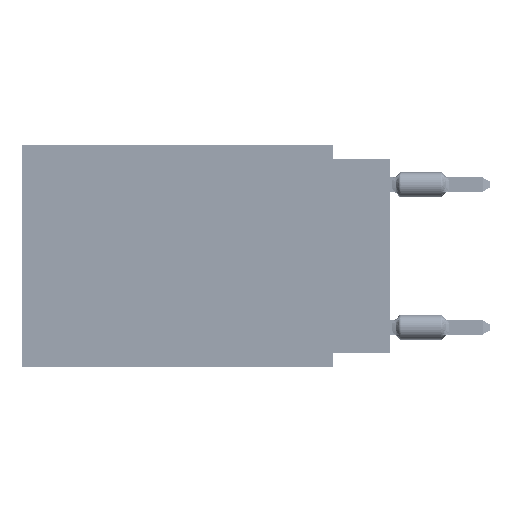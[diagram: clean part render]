
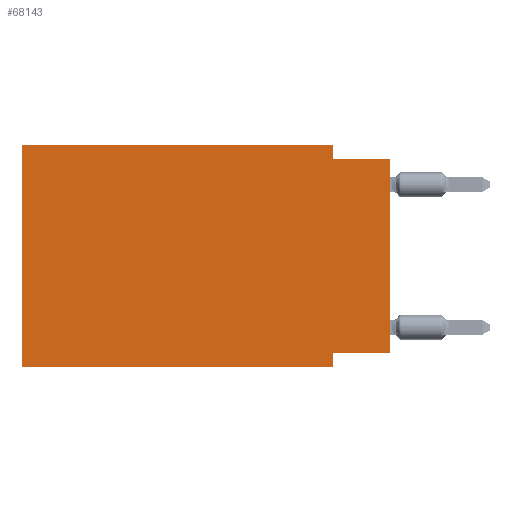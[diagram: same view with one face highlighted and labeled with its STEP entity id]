
A CAD part, left-side view. The second image highlights one B-rep face of the part: STEP entity #68143.
In plain terms, the highlighted planar face has unit normal (-1, 0, 0).
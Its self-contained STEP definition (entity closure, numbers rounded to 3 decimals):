
#1008 = CARTESIAN_POINT ( 'NONE',  ( 0., 16.383, -9.906 ) ) ;
#1446 = VERTEX_POINT ( 'NONE', #73461 ) ;
#2046 = CARTESIAN_POINT ( 'NONE',  ( 0., 16.383, 0. ) ) ;
#2713 = CARTESIAN_POINT ( 'NONE',  ( 0., 0., 0. ) ) ;
#3129 = DIRECTION ( 'NONE',  ( 0., 0., 1. ) ) ;
#3843 = EDGE_CURVE ( 'NONE', #80691, #40627, #19253, .T. ) ;
#4311 = VECTOR ( 'NONE', #3129, 1000. ) ;
#7272 = CARTESIAN_POINT ( 'NONE',  ( 0., 0., -9.271 ) ) ;
#7515 = DIRECTION ( 'NONE',  ( 0., -1., 0. ) ) ;
#8528 = VECTOR ( 'NONE', #66285, 1000. ) ;
#8894 = PLANE ( 'NONE',  #49213 ) ;
#9763 = FACE_OUTER_BOUND ( 'NONE', #35043, .T. ) ;
#11874 = EDGE_CURVE ( 'NONE', #69626, #35812, #55457, .T. ) ;
#12579 = DIRECTION ( 'NONE',  ( 0., -1., 0. ) ) ;
#13951 = LINE ( 'NONE', #33588, #33979 ) ;
#14133 = VERTEX_POINT ( 'NONE', #56360 ) ;
#15875 = CARTESIAN_POINT ( 'NONE',  ( 0., 16.383, 0. ) ) ;
#18498 = CARTESIAN_POINT ( 'NONE',  ( 0., 0., -9.271 ) ) ;
#19253 = LINE ( 'NONE', #7272, #70445 ) ;
#23016 = DIRECTION ( 'NONE',  ( 1., 0., 0. ) ) ;
#23830 = CARTESIAN_POINT ( 'NONE',  ( 0., 0., -0.635 ) ) ;
#24397 = EDGE_CURVE ( 'NONE', #40627, #78083, #77441, .T. ) ;
#24790 = CARTESIAN_POINT ( 'NONE',  ( 0., 2.54, -9.906 ) ) ;
#26283 = DIRECTION ( 'NONE',  ( 0., 0., -1. ) ) ;
#30206 = VECTOR ( 'NONE', #81484, 1000. ) ;
#30944 = ORIENTED_EDGE ( 'NONE', *, *, #80633, .T. ) ;
#30984 = CARTESIAN_POINT ( 'NONE',  ( 0., 2.54, 0. ) ) ;
#31534 = EDGE_CURVE ( 'NONE', #68642, #78083, #84329, .T. ) ;
#33588 = CARTESIAN_POINT ( 'NONE',  ( 0., 16.383, 0. ) ) ;
#33979 = VECTOR ( 'NONE', #7515, 1000. ) ;
#34979 = DIRECTION ( 'NONE',  ( 0., 0., -1. ) ) ;
#35043 = EDGE_LOOP ( 'NONE', ( #30944, #62799, #66397, #48425, #56508, #75915, #45587, #57411 ) ) ;
#35812 = VERTEX_POINT ( 'NONE', #69874 ) ;
#36823 = VECTOR ( 'NONE', #26283, 1000. ) ;
#40627 = VERTEX_POINT ( 'NONE', #73861 ) ;
#42243 = VECTOR ( 'NONE', #56142, 1000. ) ;
#45072 = LINE ( 'NONE', #30984, #36823 ) ;
#45587 = ORIENTED_EDGE ( 'NONE', *, *, #24397, .F. ) ;
#45722 = DIRECTION ( 'NONE',  ( 0., 1., 0. ) ) ;
#47055 = LINE ( 'NONE', #15875, #8528 ) ;
#48425 = ORIENTED_EDGE ( 'NONE', *, *, #66182, .F. ) ;
#49213 = AXIS2_PLACEMENT_3D ( 'NONE', #2046, #23016, #34979 ) ;
#52397 = EDGE_CURVE ( 'NONE', #68642, #14133, #47055, .T. ) ;
#54218 = CARTESIAN_POINT ( 'NONE',  ( 0., 2.54, -0.635 ) ) ;
#55457 = LINE ( 'NONE', #23830, #30206 ) ;
#55706 = LINE ( 'NONE', #2713, #4311 ) ;
#56142 = DIRECTION ( 'NONE',  ( 0., 0., -1. ) ) ;
#56360 = CARTESIAN_POINT ( 'NONE',  ( 0., 16.383, 0. ) ) ;
#56508 = ORIENTED_EDGE ( 'NONE', *, *, #52397, .F. ) ;
#57411 = ORIENTED_EDGE ( 'NONE', *, *, #3843, .F. ) ;
#62799 = ORIENTED_EDGE ( 'NONE', *, *, #11874, .F. ) ;
#64227 = CARTESIAN_POINT ( 'NONE',  ( 0., 2.54, -9.906 ) ) ;
#66182 = EDGE_CURVE ( 'NONE', #14133, #1446, #13951, .T. ) ;
#66285 = DIRECTION ( 'NONE',  ( 0., 0., 1. ) ) ;
#66397 = ORIENTED_EDGE ( 'NONE', *, *, #80416, .F. ) ;
#68143 = ADVANCED_FACE ( 'NONE', ( #9763 ), #8894, .F. ) ;
#68642 = VERTEX_POINT ( 'NONE', #75406 ) ;
#69626 = VERTEX_POINT ( 'NONE', #54218 ) ;
#69874 = CARTESIAN_POINT ( 'NONE',  ( 0., 0., -0.635 ) ) ;
#70445 = VECTOR ( 'NONE', #45722, 1000. ) ;
#73461 = CARTESIAN_POINT ( 'NONE',  ( 0., 2.54, 0. ) ) ;
#73861 = CARTESIAN_POINT ( 'NONE',  ( 0., 2.54, -9.271 ) ) ;
#75406 = CARTESIAN_POINT ( 'NONE',  ( 0., 16.383, -9.906 ) ) ;
#75915 = ORIENTED_EDGE ( 'NONE', *, *, #31534, .T. ) ;
#77441 = LINE ( 'NONE', #64227, #42243 ) ;
#77965 = VECTOR ( 'NONE', #12579, 1000. ) ;
#78083 = VERTEX_POINT ( 'NONE', #24790 ) ;
#80416 = EDGE_CURVE ( 'NONE', #1446, #69626, #45072, .T. ) ;
#80633 = EDGE_CURVE ( 'NONE', #80691, #35812, #55706, .T. ) ;
#80691 = VERTEX_POINT ( 'NONE', #18498 ) ;
#81484 = DIRECTION ( 'NONE',  ( 0., -1., 0. ) ) ;
#84329 = LINE ( 'NONE', #1008, #77965 ) ;
